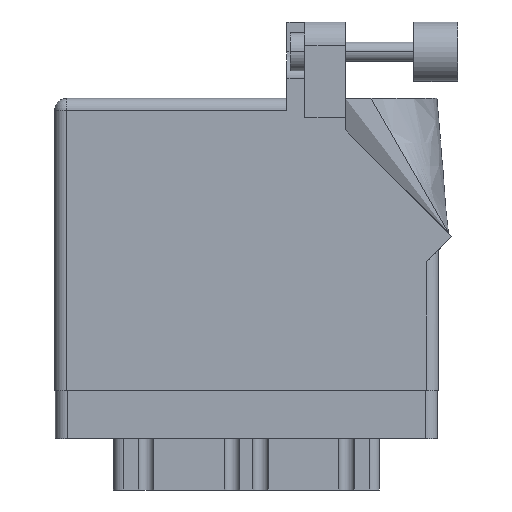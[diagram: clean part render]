
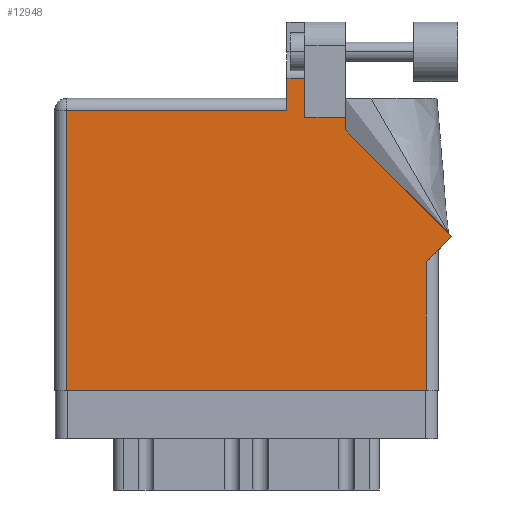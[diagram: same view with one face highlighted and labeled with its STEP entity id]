
A CAD part, front view. The second image highlights one B-rep face of the part: STEP entity #12948.
In plain terms, the highlighted face is planar.
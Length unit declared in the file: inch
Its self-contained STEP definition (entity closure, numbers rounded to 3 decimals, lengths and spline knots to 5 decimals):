
#898 = VECTOR ( 'NONE', #28106, 39.37008 ) ;
#1297 = LINE ( 'NONE', #14768, #9210 ) ;
#1508 = CARTESIAN_POINT ( 'NONE',  ( 1.311, 1.43, 0. ) ) ;
#1885 = VECTOR ( 'NONE', #24797, 39.37008 ) ;
#2609 = DIRECTION ( 'NONE',  ( 0., 0., -1. ) ) ;
#2796 = CARTESIAN_POINT ( 'NONE',  ( 0.062, 1.468, 0. ) ) ;
#3131 = CARTESIAN_POINT ( 'NONE',  ( 0., 1.53, 0. ) ) ;
#3677 = VERTEX_POINT ( 'NONE', #26925 ) ;
#4022 = LINE ( 'NONE', #33929, #898 ) ;
#4416 = CARTESIAN_POINT ( 'NONE',  ( 0.062, 0., 0. ) ) ;
#4419 = VECTOR ( 'NONE', #30473, 39.37008 ) ;
#5256 = EDGE_CURVE ( 'NONE', #18417, #14502, #14617, .T. ) ;
#5435 = ORIENTED_EDGE ( 'NONE', *, *, #8545, .T. ) ;
#6899 = VECTOR ( 'NONE', #29497, 39.37008 ) ;
#6917 = EDGE_CURVE ( 'NONE', #17356, #17786, #16886, .T. ) ;
#7543 = LINE ( 'NONE', #18338, #6899 ) ;
#7872 = EDGE_CURVE ( 'NONE', #3677, #27563, #4022, .T. ) ;
#8171 = CARTESIAN_POINT ( 'NONE',  ( 1.217, 1.468, 0. ) ) ;
#8459 = FACE_OUTER_BOUND ( 'NONE', #10562, .T. ) ;
#8545 = EDGE_CURVE ( 'NONE', #22605, #3677, #19319, .T. ) ;
#9210 = VECTOR ( 'NONE', #20048, 39.37008 ) ;
#9256 = CARTESIAN_POINT ( 'NONE',  ( 1.64177, 1.6315, 0. ) ) ;
#10375 = ORIENTED_EDGE ( 'NONE', *, *, #24432, .T. ) ;
#10562 = EDGE_LOOP ( 'NONE', ( #34619, #12168, #15724, #32223, #10375, #24709, #14332, #5435, #10601, #23451, #26813 ) ) ;
#10601 = ORIENTED_EDGE ( 'NONE', *, *, #7872, .T. ) ;
#10693 = VECTOR ( 'NONE', #15460, 39.37008 ) ;
#10914 = CARTESIAN_POINT ( 'NONE',  ( 1.311, 1.6315, 0. ) ) ;
#11356 = CARTESIAN_POINT ( 'NONE',  ( 1.524, 1.36442, 0. ) ) ;
#11912 = LINE ( 'NONE', #24999, #13919 ) ;
#12168 = ORIENTED_EDGE ( 'NONE', *, *, #6917, .T. ) ;
#12934 = VECTOR ( 'NONE', #33539, 39.37008 ) ;
#12948 = ADVANCED_FACE ( 'NONE', ( #8459 ), #19251, .F. ) ;
#13356 = VECTOR ( 'NONE', #19516, 39.37008 ) ;
#13919 = VECTOR ( 'NONE', #25349, 39.37008 ) ;
#14197 = CARTESIAN_POINT ( 'NONE',  ( 2.01, 0.737, 0. ) ) ;
#14332 = ORIENTED_EDGE ( 'NONE', *, *, #26571, .T. ) ;
#14374 = CARTESIAN_POINT ( 'NONE',  ( 1.948, 0., 0. ) ) ;
#14422 = VERTEX_POINT ( 'NONE', #33792 ) ;
#14435 = CARTESIAN_POINT ( 'NONE',  ( 0., 1.468, 0. ) ) ;
#14502 = VERTEX_POINT ( 'NONE', #2796 ) ;
#14617 = LINE ( 'NONE', #14435, #12934 ) ;
#14768 = CARTESIAN_POINT ( 'NONE',  ( 1.311, 1.43, 0. ) ) ;
#14889 = EDGE_CURVE ( 'NONE', #14422, #28550, #7543, .T. ) ;
#15460 = DIRECTION ( 'NONE',  ( 0., -1., 0. ) ) ;
#15602 = VERTEX_POINT ( 'NONE', #4416 ) ;
#15724 = ORIENTED_EDGE ( 'NONE', *, *, #27369, .T. ) ;
#16588 = LINE ( 'NONE', #31032, #34963 ) ;
#16886 = LINE ( 'NONE', #9256, #13356 ) ;
#17356 = VERTEX_POINT ( 'NONE', #10914 ) ;
#17786 = VERTEX_POINT ( 'NONE', #20952 ) ;
#18338 = CARTESIAN_POINT ( 'NONE',  ( 1.524, 1.43, 0. ) ) ;
#18417 = VERTEX_POINT ( 'NONE', #8171 ) ;
#19251 = PLANE ( 'NONE',  #33931 ) ;
#19319 = LINE ( 'NONE', #14197, #4419 ) ;
#19516 = DIRECTION ( 'NONE',  ( -1., 0., 0. ) ) ;
#20048 = DIRECTION ( 'NONE',  ( 0., 1., 0. ) ) ;
#20691 = CARTESIAN_POINT ( 'NONE',  ( 1.948, 0.737, 0. ) ) ;
#20952 = CARTESIAN_POINT ( 'NONE',  ( 1.217, 1.6315, 0. ) ) ;
#22403 = DIRECTION ( 'NONE',  ( 1., 0., 0. ) ) ;
#22605 = VERTEX_POINT ( 'NONE', #32662 ) ;
#23392 = CARTESIAN_POINT ( 'NONE',  ( 1.217, 1.53, 0. ) ) ;
#23451 = ORIENTED_EDGE ( 'NONE', *, *, #33786, .T. ) ;
#23524 = DIRECTION ( 'NONE',  ( 0., 1., 0. ) ) ;
#23920 = CARTESIAN_POINT ( 'NONE',  ( 1.524, 1.36442, 0. ) ) ;
#24184 = VECTOR ( 'NONE', #23524, 39.37008 ) ;
#24432 = EDGE_CURVE ( 'NONE', #14502, #15602, #11912, .T. ) ;
#24709 = ORIENTED_EDGE ( 'NONE', *, *, #27236, .T. ) ;
#24797 = DIRECTION ( 'NONE',  ( 0., 1., 0. ) ) ;
#24999 = CARTESIAN_POINT ( 'NONE',  ( 0.062, 0., 0. ) ) ;
#25349 = DIRECTION ( 'NONE',  ( 0., -1., 0. ) ) ;
#26571 = EDGE_CURVE ( 'NONE', #27621, #22605, #34158, .T. ) ;
#26813 = ORIENTED_EDGE ( 'NONE', *, *, #14889, .T. ) ;
#26925 = CARTESIAN_POINT ( 'NONE',  ( 2.08071, 0.80771, 0. ) ) ;
#27219 = DIRECTION ( 'NONE',  ( -1., 0., 0. ) ) ;
#27236 = EDGE_CURVE ( 'NONE', #15602, #27621, #16588, .T. ) ;
#27369 = EDGE_CURVE ( 'NONE', #17786, #18417, #33854, .T. ) ;
#27563 = VERTEX_POINT ( 'NONE', #23920 ) ;
#27621 = VERTEX_POINT ( 'NONE', #14374 ) ;
#28106 = DIRECTION ( 'NONE',  ( -0.707, 0.707, 0. ) ) ;
#28550 = VERTEX_POINT ( 'NONE', #1508 ) ;
#29497 = DIRECTION ( 'NONE',  ( -1., 0., 0. ) ) ;
#30473 = DIRECTION ( 'NONE',  ( 0.707, 0.707, 0. ) ) ;
#31032 = CARTESIAN_POINT ( 'NONE',  ( 0., 0., 0. ) ) ;
#32223 = ORIENTED_EDGE ( 'NONE', *, *, #5256, .T. ) ;
#32662 = CARTESIAN_POINT ( 'NONE',  ( 1.948, 0.675, 0. ) ) ;
#32783 = EDGE_CURVE ( 'NONE', #28550, #17356, #1297, .T. ) ;
#33463 = LINE ( 'NONE', #11356, #1885 ) ;
#33539 = DIRECTION ( 'NONE',  ( -1., 0., 0. ) ) ;
#33786 = EDGE_CURVE ( 'NONE', #27563, #14422, #33463, .T. ) ;
#33792 = CARTESIAN_POINT ( 'NONE',  ( 1.524, 1.43, 0. ) ) ;
#33854 = LINE ( 'NONE', #23392, #10693 ) ;
#33929 = CARTESIAN_POINT ( 'NONE',  ( 2.08071, 0.80771, 0. ) ) ;
#33931 = AXIS2_PLACEMENT_3D ( 'NONE', #3131, #2609, #27219 ) ;
#34158 = LINE ( 'NONE', #20691, #24184 ) ;
#34619 = ORIENTED_EDGE ( 'NONE', *, *, #32783, .T. ) ;
#34963 = VECTOR ( 'NONE', #22403, 39.37008 ) ;
